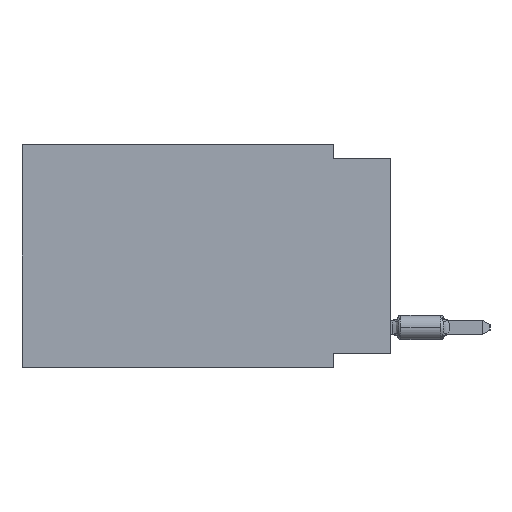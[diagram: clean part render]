
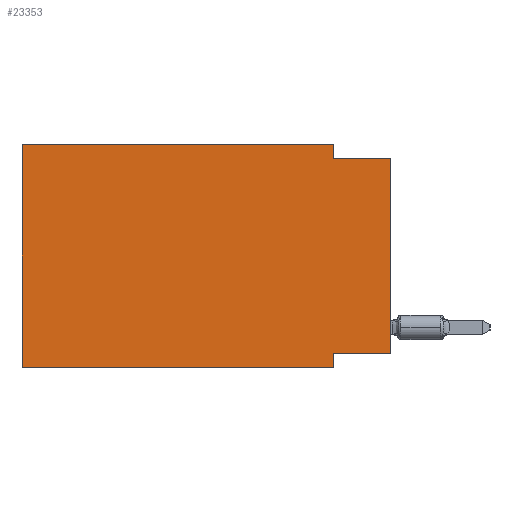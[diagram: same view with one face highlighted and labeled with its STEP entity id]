
A CAD part, left-side view. The second image highlights one B-rep face of the part: STEP entity #23353.
In plain terms, the highlighted planar face has unit normal (-1, 0, 0).
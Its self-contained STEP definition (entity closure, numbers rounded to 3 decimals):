
#35 = DIRECTION ( 'NONE',  ( 0., 0., -1. ) ) ;
#152 = EDGE_CURVE ( 'NONE', #15302, #24657, #4254, .T. ) ;
#181 = LINE ( 'NONE', #16571, #9737 ) ;
#683 = CARTESIAN_POINT ( 'NONE',  ( 0., 2.54, -0.635 ) ) ;
#1000 = ORIENTED_EDGE ( 'NONE', *, *, #14628, .T. ) ;
#1751 = VERTEX_POINT ( 'NONE', #7389 ) ;
#1827 = EDGE_CURVE ( 'NONE', #14842, #14479, #5049, .T. ) ;
#2050 = DIRECTION ( 'NONE',  ( 0., -1., 0. ) ) ;
#2273 = CARTESIAN_POINT ( 'NONE',  ( 0., 16.383, 0. ) ) ;
#2735 = DIRECTION ( 'NONE',  ( 0., -1., 0. ) ) ;
#4254 = LINE ( 'NONE', #11378, #27437 ) ;
#4541 = ORIENTED_EDGE ( 'NONE', *, *, #152, .F. ) ;
#5049 = LINE ( 'NONE', #2273, #27019 ) ;
#5416 = LINE ( 'NONE', #7730, #19403 ) ;
#6564 = ORIENTED_EDGE ( 'NONE', *, *, #1827, .F. ) ;
#6597 = LINE ( 'NONE', #8476, #28029 ) ;
#7389 = CARTESIAN_POINT ( 'NONE',  ( 0., 0., -9.271 ) ) ;
#7730 = CARTESIAN_POINT ( 'NONE',  ( 0., 0., 0. ) ) ;
#8146 = ORIENTED_EDGE ( 'NONE', *, *, #27362, .F. ) ;
#8476 = CARTESIAN_POINT ( 'NONE',  ( 0., 16.383, 0. ) ) ;
#8527 = LINE ( 'NONE', #17814, #14057 ) ;
#8678 = AXIS2_PLACEMENT_3D ( 'NONE', #12390, #23990, #35 ) ;
#8989 = CARTESIAN_POINT ( 'NONE',  ( 0., 0., -0.635 ) ) ;
#9579 = CARTESIAN_POINT ( 'NONE',  ( 0., 2.54, 0. ) ) ;
#9737 = VECTOR ( 'NONE', #2050, 1000. ) ;
#10394 = VERTEX_POINT ( 'NONE', #12136 ) ;
#11154 = EDGE_CURVE ( 'NONE', #14479, #14162, #23215, .T. ) ;
#11378 = CARTESIAN_POINT ( 'NONE',  ( 0., 2.54, -9.906 ) ) ;
#12135 = CARTESIAN_POINT ( 'NONE',  ( 0., 2.54, -9.271 ) ) ;
#12136 = CARTESIAN_POINT ( 'NONE',  ( 0., 16.383, -9.906 ) ) ;
#12250 = FACE_OUTER_BOUND ( 'NONE', #12875, .T. ) ;
#12390 = CARTESIAN_POINT ( 'NONE',  ( 0., 16.383, 0. ) ) ;
#12400 = ORIENTED_EDGE ( 'NONE', *, *, #22656, .F. ) ;
#12875 = EDGE_LOOP ( 'NONE', ( #1000, #8146, #23608, #6564, #24116, #23385, #4541, #12400 ) ) ;
#13005 = EDGE_CURVE ( 'NONE', #10394, #24657, #181, .T. ) ;
#13619 = VECTOR ( 'NONE', #18649, 1000. ) ;
#14019 = DIRECTION ( 'NONE',  ( 0., 1., 0. ) ) ;
#14057 = VECTOR ( 'NONE', #14019, 1000. ) ;
#14162 = VERTEX_POINT ( 'NONE', #683 ) ;
#14186 = CARTESIAN_POINT ( 'NONE',  ( 0., 16.383, 0. ) ) ;
#14404 = CARTESIAN_POINT ( 'NONE',  ( 0., 2.54, -9.906 ) ) ;
#14479 = VERTEX_POINT ( 'NONE', #9579 ) ;
#14628 = EDGE_CURVE ( 'NONE', #1751, #23288, #5416, .T. ) ;
#14842 = VERTEX_POINT ( 'NONE', #14186 ) ;
#15302 = VERTEX_POINT ( 'NONE', #12135 ) ;
#16571 = CARTESIAN_POINT ( 'NONE',  ( 0., 16.383, -9.906 ) ) ;
#17162 = DIRECTION ( 'NONE',  ( 0., 0., 1. ) ) ;
#17814 = CARTESIAN_POINT ( 'NONE',  ( 0., 0., -9.271 ) ) ;
#17894 = DIRECTION ( 'NONE',  ( 0., 0., 1. ) ) ;
#17966 = VECTOR ( 'NONE', #23348, 1000. ) ;
#18649 = DIRECTION ( 'NONE',  ( 0., -1., 0. ) ) ;
#19403 = VECTOR ( 'NONE', #17162, 1000. ) ;
#20805 = DIRECTION ( 'NONE',  ( 0., 0., -1. ) ) ;
#20878 = CARTESIAN_POINT ( 'NONE',  ( 0., 2.54, 0. ) ) ;
#22656 = EDGE_CURVE ( 'NONE', #1751, #15302, #8527, .T. ) ;
#23215 = LINE ( 'NONE', #20878, #17966 ) ;
#23288 = VERTEX_POINT ( 'NONE', #8989 ) ;
#23348 = DIRECTION ( 'NONE',  ( 0., 0., -1. ) ) ;
#23353 = ADVANCED_FACE ( 'NONE', ( #12250 ), #28958, .F. ) ;
#23385 = ORIENTED_EDGE ( 'NONE', *, *, #13005, .T. ) ;
#23605 = CARTESIAN_POINT ( 'NONE',  ( 0., 0., -0.635 ) ) ;
#23608 = ORIENTED_EDGE ( 'NONE', *, *, #11154, .F. ) ;
#23990 = DIRECTION ( 'NONE',  ( 1., 0., 0. ) ) ;
#24116 = ORIENTED_EDGE ( 'NONE', *, *, #30234, .F. ) ;
#24657 = VERTEX_POINT ( 'NONE', #14404 ) ;
#27019 = VECTOR ( 'NONE', #2735, 1000. ) ;
#27362 = EDGE_CURVE ( 'NONE', #14162, #23288, #28108, .T. ) ;
#27437 = VECTOR ( 'NONE', #20805, 1000. ) ;
#28029 = VECTOR ( 'NONE', #17894, 1000. ) ;
#28108 = LINE ( 'NONE', #23605, #13619 ) ;
#28958 = PLANE ( 'NONE',  #8678 ) ;
#30234 = EDGE_CURVE ( 'NONE', #10394, #14842, #6597, .T. ) ;
